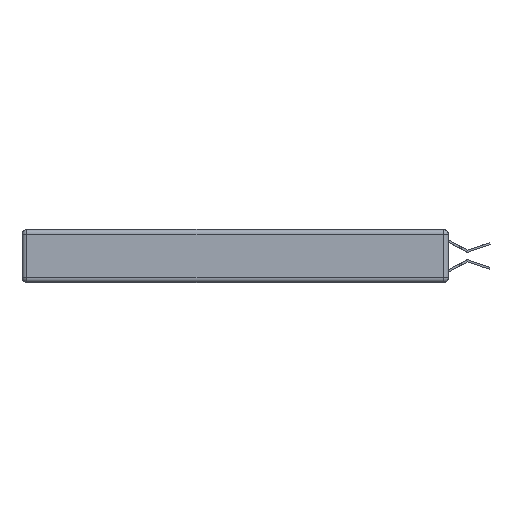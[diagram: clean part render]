
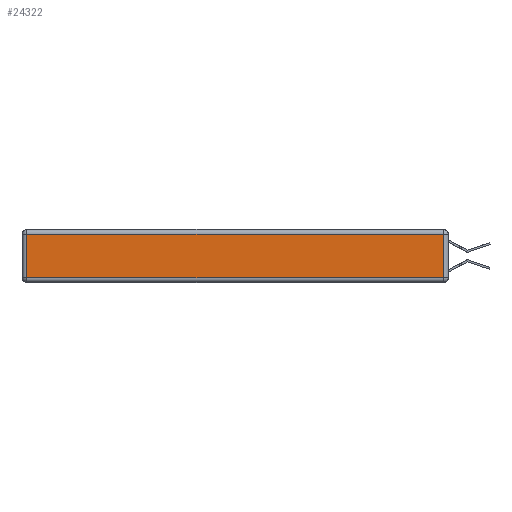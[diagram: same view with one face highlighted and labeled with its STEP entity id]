
A CAD part, left-side view. The second image highlights one B-rep face of the part: STEP entity #24322.
In plain terms, the highlighted planar face has unit normal (-1, 0, 0).
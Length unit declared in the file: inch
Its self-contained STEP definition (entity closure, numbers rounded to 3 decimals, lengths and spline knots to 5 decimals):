
#91 = LINE ( 'NONE', #25506, #26142 ) ;
#790 = VERTEX_POINT ( 'NONE', #18774 ) ;
#944 = AXIS2_PLACEMENT_3D ( 'NONE', #9652, #22676, #4963 ) ;
#2816 = CARTESIAN_POINT ( 'NONE',  ( 0., 2.72, -0.313 ) ) ;
#3241 = LINE ( 'NONE', #26868, #15579 ) ;
#3248 = ORIENTED_EDGE ( 'NONE', *, *, #16563, .T. ) ;
#3676 = VECTOR ( 'NONE', #23308, 39.37008 ) ;
#4963 = DIRECTION ( 'NONE',  ( 0., 0., 1. ) ) ;
#5981 = CARTESIAN_POINT ( 'NONE',  ( 0., 0., -0.313 ) ) ;
#8083 = FACE_OUTER_BOUND ( 'NONE', #28150, .T. ) ;
#8476 = CARTESIAN_POINT ( 'NONE',  ( 0., 0.03, -0.313 ) ) ;
#9652 = CARTESIAN_POINT ( 'NONE',  ( 0., 0., -0.343 ) ) ;
#10041 = EDGE_CURVE ( 'NONE', #11844, #790, #91, .T. ) ;
#11694 = VERTEX_POINT ( 'NONE', #2816 ) ;
#11844 = VERTEX_POINT ( 'NONE', #21095 ) ;
#11848 = VECTOR ( 'NONE', #28229, 39.37008 ) ;
#14972 = VERTEX_POINT ( 'NONE', #8476 ) ;
#15579 = VECTOR ( 'NONE', #15856, 39.37008 ) ;
#15856 = DIRECTION ( 'NONE',  ( 0., 0., 1. ) ) ;
#16171 = PLANE ( 'NONE',  #944 ) ;
#16563 = EDGE_CURVE ( 'NONE', #11694, #14972, #17376, .T. ) ;
#16598 = DIRECTION ( 'NONE',  ( 0., 1., 0. ) ) ;
#17376 = LINE ( 'NONE', #5981, #3676 ) ;
#17833 = EDGE_CURVE ( 'NONE', #790, #11694, #21056, .T. ) ;
#18774 = CARTESIAN_POINT ( 'NONE',  ( 0., 2.72, -0.03 ) ) ;
#21056 = LINE ( 'NONE', #21529, #11848 ) ;
#21095 = CARTESIAN_POINT ( 'NONE',  ( 0., 0.03, -0.03 ) ) ;
#21529 = CARTESIAN_POINT ( 'NONE',  ( 0., 2.72, -0.343 ) ) ;
#21569 = ORIENTED_EDGE ( 'NONE', *, *, #10041, .T. ) ;
#22676 = DIRECTION ( 'NONE',  ( -1., 0., 0. ) ) ;
#23308 = DIRECTION ( 'NONE',  ( 0., -1., 0. ) ) ;
#23627 = ORIENTED_EDGE ( 'NONE', *, *, #24676, .T. ) ;
#24322 = ADVANCED_FACE ( 'NONE', ( #8083 ), #16171, .T. ) ;
#24336 = ORIENTED_EDGE ( 'NONE', *, *, #17833, .T. ) ;
#24676 = EDGE_CURVE ( 'NONE', #14972, #11844, #3241, .T. ) ;
#25506 = CARTESIAN_POINT ( 'NONE',  ( 0., 2.75, -0.03 ) ) ;
#26142 = VECTOR ( 'NONE', #16598, 39.37008 ) ;
#26868 = CARTESIAN_POINT ( 'NONE',  ( 0., 0.03, -0.343 ) ) ;
#28150 = EDGE_LOOP ( 'NONE', ( #3248, #23627, #21569, #24336 ) ) ;
#28229 = DIRECTION ( 'NONE',  ( 0., 0., -1. ) ) ;
